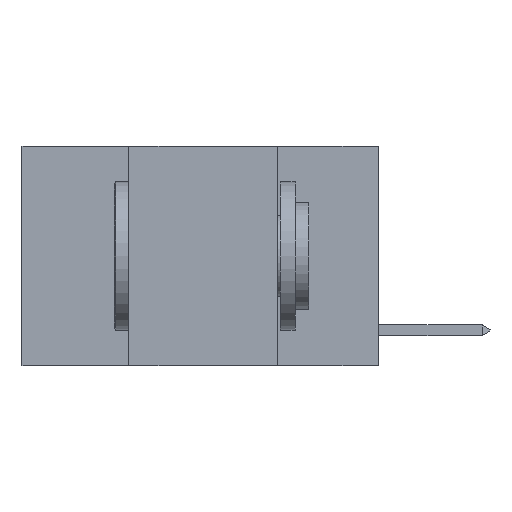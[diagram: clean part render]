
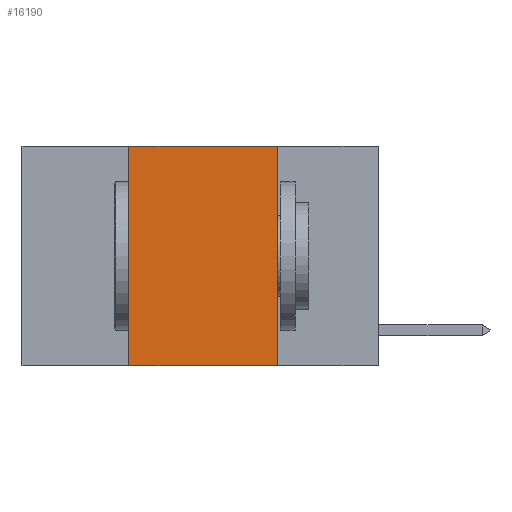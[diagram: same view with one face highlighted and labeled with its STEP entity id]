
A CAD part, left-side view. The second image highlights one B-rep face of the part: STEP entity #16190.
In plain terms, the highlighted planar face has unit normal (-1, 0, 0).
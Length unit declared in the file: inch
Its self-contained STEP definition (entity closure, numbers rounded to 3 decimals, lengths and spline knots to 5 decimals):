
#74 = CARTESIAN_POINT ( 'NONE',  ( 0., 0.42, 0. ) ) ;
#541 = CARTESIAN_POINT ( 'NONE',  ( 0., 0.17, 0. ) ) ;
#760 = CARTESIAN_POINT ( 'NONE',  ( 0., 0.42, 0. ) ) ;
#1695 = VERTEX_POINT ( 'NONE', #541 ) ;
#2918 = LINE ( 'NONE', #5101, #14031 ) ;
#4102 = VERTEX_POINT ( 'NONE', #11683 ) ;
#4618 = DIRECTION ( 'NONE',  ( 0., -1., 0. ) ) ;
#5101 = CARTESIAN_POINT ( 'NONE',  ( 0., 0.6, 0. ) ) ;
#5974 = ORIENTED_EDGE ( 'NONE', *, *, #12230, .T. ) ;
#6360 = EDGE_CURVE ( 'NONE', #1695, #6586, #10611, .T. ) ;
#6418 = DIRECTION ( 'NONE',  ( 0., 0., -1. ) ) ;
#6419 = LINE ( 'NONE', #74, #17081 ) ;
#6576 = EDGE_LOOP ( 'NONE', ( #9930, #10253, #7046, #5974 ) ) ;
#6586 = VERTEX_POINT ( 'NONE', #16905 ) ;
#6916 = EDGE_CURVE ( 'NONE', #9508, #1695, #2918, .T. ) ;
#7046 = ORIENTED_EDGE ( 'NONE', *, *, #10363, .F. ) ;
#7192 = DIRECTION ( 'NONE',  ( 0., 0., 1. ) ) ;
#8115 = LINE ( 'NONE', #17100, #15075 ) ;
#9312 = DIRECTION ( 'NONE',  ( 0., -1., 0. ) ) ;
#9508 = VERTEX_POINT ( 'NONE', #760 ) ;
#9930 = ORIENTED_EDGE ( 'NONE', *, *, #6360, .F. ) ;
#10253 = ORIENTED_EDGE ( 'NONE', *, *, #6916, .F. ) ;
#10363 = EDGE_CURVE ( 'NONE', #4102, #9508, #6419, .T. ) ;
#10611 = LINE ( 'NONE', #13630, #17536 ) ;
#11683 = CARTESIAN_POINT ( 'NONE',  ( 0., 0.42, -0.37 ) ) ;
#11978 = CARTESIAN_POINT ( 'NONE',  ( 0., 0.6, 0. ) ) ;
#12230 = EDGE_CURVE ( 'NONE', #4102, #6586, #8115, .T. ) ;
#13630 = CARTESIAN_POINT ( 'NONE',  ( 0., 0.17, 0. ) ) ;
#14031 = VECTOR ( 'NONE', #9312, 39.37008 ) ;
#14548 = AXIS2_PLACEMENT_3D ( 'NONE', #11978, #14736, #6418 ) ;
#14736 = DIRECTION ( 'NONE',  ( 1., 0., 0. ) ) ;
#15075 = VECTOR ( 'NONE', #4618, 39.37008 ) ;
#16190 = ADVANCED_FACE ( 'NONE', ( #16271 ), #17471, .F. ) ;
#16271 = FACE_OUTER_BOUND ( 'NONE', #6576, .T. ) ;
#16424 = DIRECTION ( 'NONE',  ( 0., 0., -1. ) ) ;
#16905 = CARTESIAN_POINT ( 'NONE',  ( 0., 0.17, -0.37 ) ) ;
#17081 = VECTOR ( 'NONE', #7192, 39.37008 ) ;
#17100 = CARTESIAN_POINT ( 'NONE',  ( 0., 0.6, -0.37 ) ) ;
#17471 = PLANE ( 'NONE',  #14548 ) ;
#17536 = VECTOR ( 'NONE', #16424, 39.37008 ) ;
